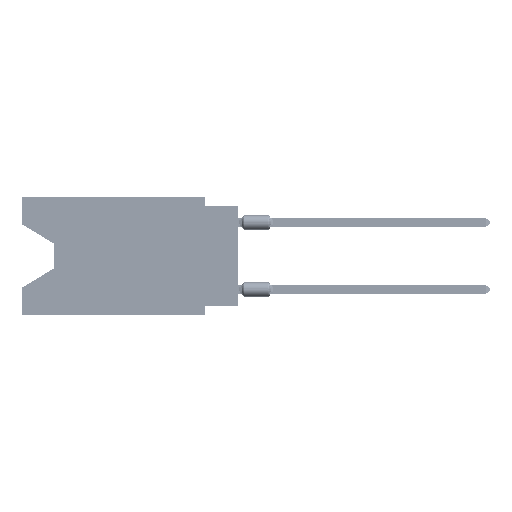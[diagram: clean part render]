
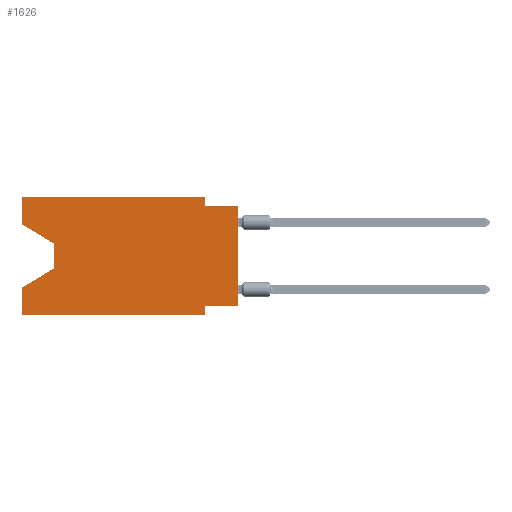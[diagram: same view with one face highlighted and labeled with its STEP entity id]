
A CAD part, left-side view. The second image highlights one B-rep face of the part: STEP entity #1626.
In plain terms, the highlighted planar face has unit normal (-1, 0, 0).
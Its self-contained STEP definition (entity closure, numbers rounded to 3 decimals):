
#1624 = LINE ( 'NONE', #8499, #53494 ) ;
#1626 = ADVANCED_FACE ( 'NONE', ( #69109 ), #82771, .F. ) ;
#1801 = ORIENTED_EDGE ( 'NONE', *, *, #10282, .F. ) ;
#2043 = DIRECTION ( 'NONE',  ( 0., 0.855, -0.519 ) ) ;
#3698 = LINE ( 'NONE', #74777, #47632 ) ;
#3999 = VECTOR ( 'NONE', #47025, 1000. ) ;
#5841 = VERTEX_POINT ( 'NONE', #71497 ) ;
#7800 = VECTOR ( 'NONE', #11808, 1000. ) ;
#7979 = VERTEX_POINT ( 'NONE', #79178 ) ;
#8499 = CARTESIAN_POINT ( 'NONE',  ( 0., 13.97, -5.385 ) ) ;
#8506 = EDGE_CURVE ( 'NONE', #24405, #26180, #55939, .T. ) ;
#9099 = CARTESIAN_POINT ( 'NONE',  ( 0., 2.54, -0.635 ) ) ;
#9398 = CARTESIAN_POINT ( 'NONE',  ( 0., 2.54, 0. ) ) ;
#9835 = EDGE_LOOP ( 'NONE', ( #83024, #63344, #28664, #43036, #12582, #1801, #18129, #34914, #61436, #76295, #81819, #73347 ) ) ;
#10282 = EDGE_CURVE ( 'NONE', #26180, #76168, #75110, .T. ) ;
#10826 = LINE ( 'NONE', #36945, #74082 ) ;
#11329 = VERTEX_POINT ( 'NONE', #67012 ) ;
#11808 = DIRECTION ( 'NONE',  ( 0., 0., 1. ) ) ;
#12582 = ORIENTED_EDGE ( 'NONE', *, *, #50947, .T. ) ;
#12984 = VECTOR ( 'NONE', #70789, 1000. ) ;
#13345 = AXIS2_PLACEMENT_3D ( 'NONE', #17705, #43394, #55833 ) ;
#13899 = CARTESIAN_POINT ( 'NONE',  ( 0., 16.383, 0. ) ) ;
#15261 = DIRECTION ( 'NONE',  ( 0., 1., 0. ) ) ;
#16256 = VERTEX_POINT ( 'NONE', #66328 ) ;
#17705 = CARTESIAN_POINT ( 'NONE',  ( 0., 16.383, 0. ) ) ;
#18129 = ORIENTED_EDGE ( 'NONE', *, *, #8506, .F. ) ;
#18141 = CARTESIAN_POINT ( 'NONE',  ( 0., 2.54, -8.89 ) ) ;
#18231 = CARTESIAN_POINT ( 'NONE',  ( 0., 0., 0. ) ) ;
#18268 = VERTEX_POINT ( 'NONE', #13899 ) ;
#18332 = CARTESIAN_POINT ( 'NONE',  ( 0., 16.383, 0. ) ) ;
#21709 = DIRECTION ( 'NONE',  ( 0., -1., 0. ) ) ;
#22896 = VECTOR ( 'NONE', #21709, 1000. ) ;
#24405 = VERTEX_POINT ( 'NONE', #62855 ) ;
#26180 = VERTEX_POINT ( 'NONE', #82443 ) ;
#26286 = VECTOR ( 'NONE', #67641, 1000. ) ;
#26447 = CARTESIAN_POINT ( 'NONE',  ( 0., 16.383, 0. ) ) ;
#27323 = CARTESIAN_POINT ( 'NONE',  ( 0., 16.383, -6.852 ) ) ;
#27913 = EDGE_CURVE ( 'NONE', #16256, #58391, #41925, .T. ) ;
#28664 = ORIENTED_EDGE ( 'NONE', *, *, #39990, .T. ) ;
#29277 = CARTESIAN_POINT ( 'NONE',  ( 0., 16.383, 0. ) ) ;
#34914 = ORIENTED_EDGE ( 'NONE', *, *, #73502, .T. ) ;
#35344 = CARTESIAN_POINT ( 'NONE',  ( 0., 0., -0.635 ) ) ;
#36562 = DIRECTION ( 'NONE',  ( 0., 0., 1. ) ) ;
#36945 = CARTESIAN_POINT ( 'NONE',  ( 0., 0., -0.635 ) ) ;
#37171 = EDGE_CURVE ( 'NONE', #7979, #61976, #54720, .T. ) ;
#39990 = EDGE_CURVE ( 'NONE', #61976, #79442, #1624, .T. ) ;
#41925 = LINE ( 'NONE', #9398, #26286 ) ;
#43036 = ORIENTED_EDGE ( 'NONE', *, *, #64957, .F. ) ;
#43083 = CARTESIAN_POINT ( 'NONE',  ( 0., 0., -8.255 ) ) ;
#43394 = DIRECTION ( 'NONE',  ( 1., 0., 0. ) ) ;
#43720 = CARTESIAN_POINT ( 'NONE',  ( 0., 13.97, -5.385 ) ) ;
#45752 = LINE ( 'NONE', #78719, #3999 ) ;
#47025 = DIRECTION ( 'NONE',  ( 0., -1., 0. ) ) ;
#47401 = LINE ( 'NONE', #26447, #22896 ) ;
#47632 = VECTOR ( 'NONE', #55948, 1000. ) ;
#50947 = EDGE_CURVE ( 'NONE', #5841, #76168, #45752, .T. ) ;
#53494 = VECTOR ( 'NONE', #2043, 1000. ) ;
#54591 = EDGE_CURVE ( 'NONE', #58391, #79975, #10826, .T. ) ;
#54720 = LINE ( 'NONE', #69282, #67015 ) ;
#55556 = VECTOR ( 'NONE', #36562, 1000. ) ;
#55833 = DIRECTION ( 'NONE',  ( 0., 0., -1. ) ) ;
#55939 = LINE ( 'NONE', #43083, #66055 ) ;
#55948 = DIRECTION ( 'NONE',  ( 0., -0.855, -0.519 ) ) ;
#56692 = CARTESIAN_POINT ( 'NONE',  ( 0., 2.54, -8.89 ) ) ;
#57615 = LINE ( 'NONE', #18231, #7800 ) ;
#58391 = VERTEX_POINT ( 'NONE', #9099 ) ;
#61359 = EDGE_CURVE ( 'NONE', #11329, #18268, #74240, .T. ) ;
#61436 = ORIENTED_EDGE ( 'NONE', *, *, #54591, .F. ) ;
#61976 = VERTEX_POINT ( 'NONE', #43720 ) ;
#62254 = EDGE_CURVE ( 'NONE', #11329, #7979, #3698, .T. ) ;
#62855 = CARTESIAN_POINT ( 'NONE',  ( 0., 0., -8.255 ) ) ;
#63344 = ORIENTED_EDGE ( 'NONE', *, *, #37171, .T. ) ;
#64957 = EDGE_CURVE ( 'NONE', #5841, #79442, #83405, .T. ) ;
#66055 = VECTOR ( 'NONE', #15261, 1000. ) ;
#66328 = CARTESIAN_POINT ( 'NONE',  ( 0., 2.54, 0. ) ) ;
#67012 = CARTESIAN_POINT ( 'NONE',  ( 0., 16.383, -2.038 ) ) ;
#67015 = VECTOR ( 'NONE', #75708, 1000. ) ;
#67641 = DIRECTION ( 'NONE',  ( 0., 0., -1. ) ) ;
#68909 = DIRECTION ( 'NONE',  ( 0., 0., 1. ) ) ;
#69109 = FACE_OUTER_BOUND ( 'NONE', #9835, .T. ) ;
#69282 = CARTESIAN_POINT ( 'NONE',  ( 0., 13.97, -3.505 ) ) ;
#70335 = DIRECTION ( 'NONE',  ( 0., -1., 0. ) ) ;
#70789 = DIRECTION ( 'NONE',  ( 0., 0., -1. ) ) ;
#70985 = VECTOR ( 'NONE', #68909, 1000. ) ;
#71497 = CARTESIAN_POINT ( 'NONE',  ( 0., 16.383, -8.89 ) ) ;
#73347 = ORIENTED_EDGE ( 'NONE', *, *, #61359, .F. ) ;
#73502 = EDGE_CURVE ( 'NONE', #24405, #79975, #57615, .T. ) ;
#74082 = VECTOR ( 'NONE', #70335, 1000. ) ;
#74240 = LINE ( 'NONE', #29277, #55556 ) ;
#74777 = CARTESIAN_POINT ( 'NONE',  ( 0., 16.383, -2.038 ) ) ;
#75110 = LINE ( 'NONE', #56692, #12984 ) ;
#75476 = EDGE_CURVE ( 'NONE', #18268, #16256, #47401, .T. ) ;
#75708 = DIRECTION ( 'NONE',  ( 0., 0., -1. ) ) ;
#76168 = VERTEX_POINT ( 'NONE', #18141 ) ;
#76295 = ORIENTED_EDGE ( 'NONE', *, *, #27913, .F. ) ;
#78719 = CARTESIAN_POINT ( 'NONE',  ( 0., 16.383, -8.89 ) ) ;
#79178 = CARTESIAN_POINT ( 'NONE',  ( 0., 13.97, -3.505 ) ) ;
#79442 = VERTEX_POINT ( 'NONE', #27323 ) ;
#79975 = VERTEX_POINT ( 'NONE', #35344 ) ;
#81819 = ORIENTED_EDGE ( 'NONE', *, *, #75476, .F. ) ;
#82443 = CARTESIAN_POINT ( 'NONE',  ( 0., 2.54, -8.255 ) ) ;
#82771 = PLANE ( 'NONE',  #13345 ) ;
#83024 = ORIENTED_EDGE ( 'NONE', *, *, #62254, .T. ) ;
#83405 = LINE ( 'NONE', #18332, #70985 ) ;
